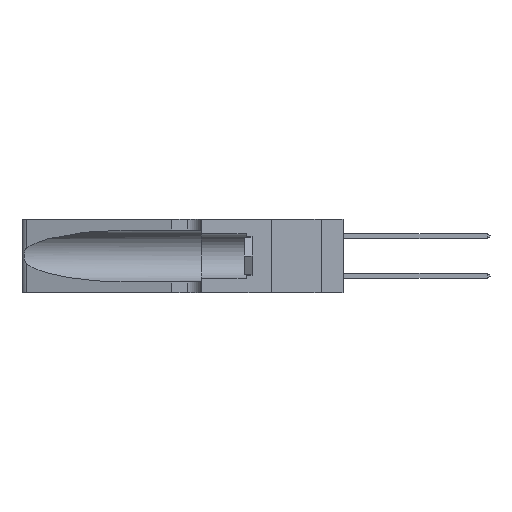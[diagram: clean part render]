
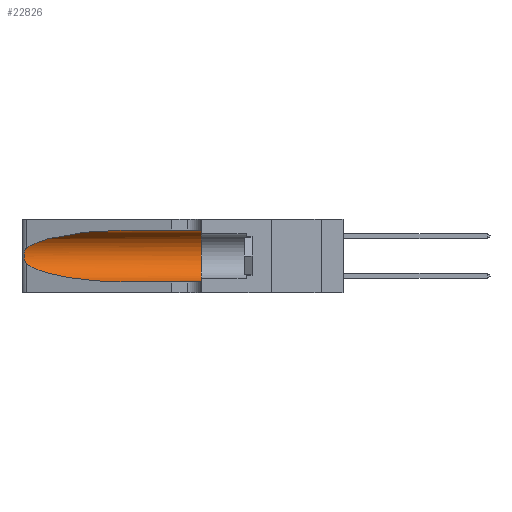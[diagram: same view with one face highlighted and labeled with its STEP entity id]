
A CAD part, left-side view. The second image highlights one B-rep face of the part: STEP entity #22826.
In plain terms, the highlighted cylindrical face has radius 3.308 mm (diameter 6.617 mm), a partial arc.
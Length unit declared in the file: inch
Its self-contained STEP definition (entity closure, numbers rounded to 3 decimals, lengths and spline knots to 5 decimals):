
#538 = ORIENTED_EDGE ( 'NONE', *, *, #18850, .F. ) ;
#746 = CARTESIAN_POINT ( 'NONE',  ( 0.1305, 0.35, 0.05475 ) ) ;
#1074 = VERTEX_POINT ( 'NONE', #34719 ) ;
#2142 = EDGE_CURVE ( 'NONE', #22444, #1074, #11441, .T. ) ;
#2182 = CARTESIAN_POINT ( 'NONE',  ( 0.25487, 1.22718, 0.22369 ) ) ;
#2303 = CARTESIAN_POINT ( 'NONE',  ( 0.25789, 1.23486, 0.15765 ) ) ;
#2703 = DIRECTION ( 'NONE',  ( 0., 0., -1. ) ) ;
#2985 = CARTESIAN_POINT ( 'NONE',  ( 0.1305, 1.61858, 0.31525 ) ) ;
#3228 = CARTESIAN_POINT ( 'NONE',  ( 0.25487, 1.22718, 0.14631 ) ) ;
#4141 = VERTEX_POINT ( 'NONE', #11987 ) ;
#5165 = CARTESIAN_POINT ( 'NONE',  ( 0.25555, 1.22993, 0.14849 ) ) ;
#5246 = CARTESIAN_POINT ( 'NONE',  ( 0.25487, 1.22718, 0.14631 ) ) ;
#7594 = CARTESIAN_POINT ( 'NONE',  ( 0.18966, 0.96281, 0.31525 ) ) ;
#7624 = ORIENTED_EDGE ( 'NONE', *, *, #10294, .T. ) ;
#8150 = CARTESIAN_POINT ( 'NONE',  ( 0.18966, 0.96281, 0.05475 ) ) ;
#10294 = EDGE_CURVE ( 'NONE', #1074, #36428, #30088, .T. ) ;
#10830 = CARTESIAN_POINT ( 'NONE',  ( 0.25787, 1.23484, 0.2124 ) ) ;
#11441 =( BOUNDED_CURVE ( )  B_SPLINE_CURVE ( 3, ( #5246, #25018, #8150, #27816 ),
 .UNSPECIFIED., .F., .T. ) 
 B_SPLINE_CURVE_WITH_KNOTS ( ( 4, 4 ),
 ( 3.44316, 4.71239 ),
 .UNSPECIFIED. ) 
 CURVE ( )  GEOMETRIC_REPRESENTATION_ITEM ( )  RATIONAL_B_SPLINE_CURVE ( ( 1., 0.87, 0.87, 1. ) ) 
 REPRESENTATION_ITEM ( '' )  );
#11987 = CARTESIAN_POINT ( 'NONE',  ( 0.25487, 1.22718, 0.22369 ) ) ;
#12011 = CARTESIAN_POINT ( 'NONE',  ( 0.1305, 0.35, 0.31525 ) ) ;
#12130 = DIRECTION ( 'NONE',  ( 0., -1., 0. ) ) ;
#12558 =( BOUNDED_CURVE ( )  B_SPLINE_CURVE ( 3, ( #27289, #7594, #30103, #13342 ),
 .UNSPECIFIED., .F., .T. ) 
 B_SPLINE_CURVE_WITH_KNOTS ( ( 4, 4 ),
 ( 1.5708, 2.84003 ),
 .UNSPECIFIED. ) 
 CURVE ( )  GEOMETRIC_REPRESENTATION_ITEM ( )  RATIONAL_B_SPLINE_CURVE ( ( 1., 0.87, 0.87, 1. ) ) 
 REPRESENTATION_ITEM ( '' )  );
#12972 = VECTOR ( 'NONE', #31106, 39.37008 ) ;
#13342 = CARTESIAN_POINT ( 'NONE',  ( 0.25487, 1.22718, 0.22369 ) ) ;
#13391 = ORIENTED_EDGE ( 'NONE', *, *, #2142, .T. ) ;
#13664 = CARTESIAN_POINT ( 'NONE',  ( 0.26018, 1.23835, 0.19895 ) ) ;
#13872 = LINE ( 'NONE', #2985, #12972 ) ;
#14932 = DIRECTION ( 'NONE',  ( 0., 1., 0. ) ) ;
#16482 = CARTESIAN_POINT ( 'NONE',  ( 0.26075, 1.23896, 0.178 ) ) ;
#16968 = EDGE_CURVE ( 'NONE', #4141, #22444, #28272, .T. ) ;
#17729 = CYLINDRICAL_SURFACE ( 'NONE', #18615, 0.13025 ) ;
#17849 = VECTOR ( 'NONE', #12130, 39.37008 ) ;
#18610 = FACE_OUTER_BOUND ( 'NONE', #28049, .T. ) ;
#18615 = AXIS2_PLACEMENT_3D ( 'NONE', #36439, #19723, #2703 ) ;
#18832 = VERTEX_POINT ( 'NONE', #12011 ) ;
#18850 = EDGE_CURVE ( 'NONE', #18832, #36428, #33728, .T. ) ;
#19197 = CARTESIAN_POINT ( 'NONE',  ( 0.25555, 1.22994, 0.2215 ) ) ;
#19321 = CARTESIAN_POINT ( 'NONE',  ( 0.25856, 1.23593, 0.16098 ) ) ;
#19723 = DIRECTION ( 'NONE',  ( 0., -1., 0. ) ) ;
#20098 = ORIENTED_EDGE ( 'NONE', *, *, #16968, .T. ) ;
#20748 = EDGE_CURVE ( 'NONE', #23897, #18832, #13872, .T. ) ;
#21358 = AXIS2_PLACEMENT_3D ( 'NONE', #31714, #14932, #34518 ) ;
#22164 = CARTESIAN_POINT ( 'NONE',  ( 0.25639, 1.23186, 0.15144 ) ) ;
#22444 = VERTEX_POINT ( 'NONE', #3228 ) ;
#22826 = ADVANCED_FACE ( 'NONE', ( #18610 ), #17729, .F. ) ;
#23239 = ORIENTED_EDGE ( 'NONE', *, *, #32970, .T. ) ;
#23897 = VERTEX_POINT ( 'NONE', #26716 ) ;
#24843 = ORIENTED_EDGE ( 'NONE', *, *, #20748, .F. ) ;
#24933 = CARTESIAN_POINT ( 'NONE',  ( 0.25487, 1.22718, 0.14631 ) ) ;
#25018 = CARTESIAN_POINT ( 'NONE',  ( 0.2373, 1.15595, 0.08982 ) ) ;
#26088 = CARTESIAN_POINT ( 'NONE',  ( 0.1305, 1.61858, 0.05475 ) ) ;
#26716 = CARTESIAN_POINT ( 'NONE',  ( 0.1305, 0.72297, 0.31525 ) ) ;
#27289 = CARTESIAN_POINT ( 'NONE',  ( 0.1305, 0.72297, 0.31525 ) ) ;
#27620 = CARTESIAN_POINT ( 'NONE',  ( 0.25639, 1.23184, 0.21858 ) ) ;
#27816 = CARTESIAN_POINT ( 'NONE',  ( 0.1305, 0.72297, 0.05475 ) ) ;
#28049 = EDGE_LOOP ( 'NONE', ( #23239, #20098, #13391, #7624, #538, #24843 ) ) ;
#28272 = B_SPLINE_CURVE_WITH_KNOTS ( 'NONE', 3,
 ( #2182, #19197, #27620, #10830, #30443, #13664, #33239, #16482, #36045, #19321, #2303, #22164, #5165, #24933 ),
 .UNSPECIFIED., .F., .F.,
 ( 4, 2, 2, 2, 2, 2, 4 ),
 ( 0., 0.00027, 0.00053, 0.00107, 0.0016, 0.00187, 0.00214 ),
 .UNSPECIFIED. ) ;
#30088 = LINE ( 'NONE', #26088, #17849 ) ;
#30103 = CARTESIAN_POINT ( 'NONE',  ( 0.2373, 1.15595, 0.28018 ) ) ;
#30443 = CARTESIAN_POINT ( 'NONE',  ( 0.25854, 1.2359, 0.20912 ) ) ;
#31106 = DIRECTION ( 'NONE',  ( 0., -1., 0. ) ) ;
#31714 = CARTESIAN_POINT ( 'NONE',  ( 0.1305, 0.35, 0.185 ) ) ;
#32970 = EDGE_CURVE ( 'NONE', #23897, #4141, #12558, .T. ) ;
#33239 = CARTESIAN_POINT ( 'NONE',  ( 0.26075, 1.23896, 0.19203 ) ) ;
#33728 = CIRCLE ( 'NONE', #21358, 0.13025 ) ;
#34518 = DIRECTION ( 'NONE',  ( 0., 0., 1. ) ) ;
#34719 = CARTESIAN_POINT ( 'NONE',  ( 0.1305, 0.72297, 0.05475 ) ) ;
#36045 = CARTESIAN_POINT ( 'NONE',  ( 0.26017, 1.23833, 0.17102 ) ) ;
#36428 = VERTEX_POINT ( 'NONE', #746 ) ;
#36439 = CARTESIAN_POINT ( 'NONE',  ( 0.1305, 1.61858, 0.185 ) ) ;
